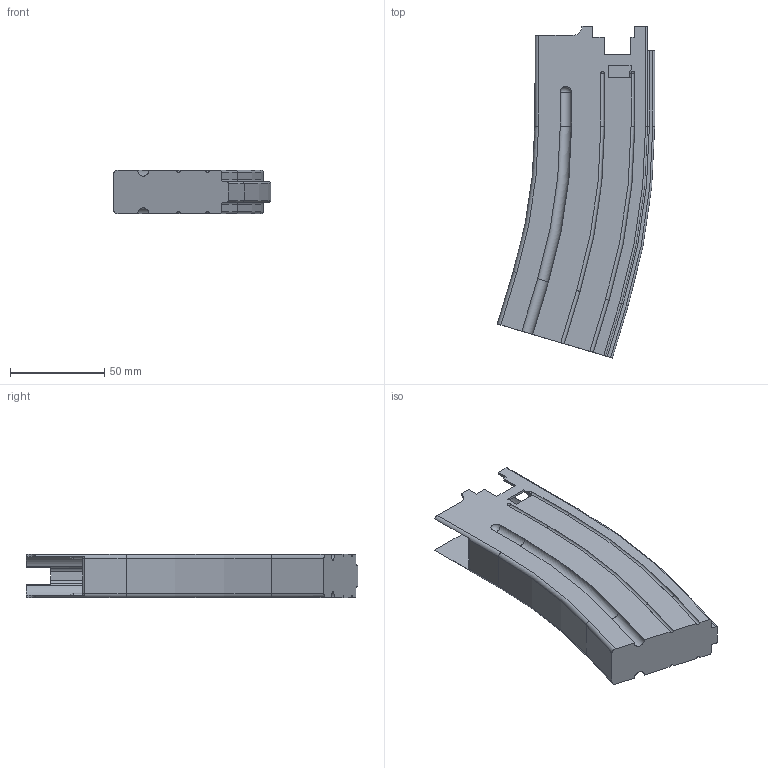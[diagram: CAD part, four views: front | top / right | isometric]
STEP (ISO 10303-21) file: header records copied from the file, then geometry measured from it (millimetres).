
FILE_DESCRIPTION (( 'STEP AP203' ), '1' );
FILE_NAME ('mag.STEP', '2021-12-29T04:18:24', ( '' ), ( '' ), 'SwSTEP 2.0', 'SolidWorks 2015', '' );
FILE_SCHEMA (( 'CONFIG_CONTROL_DESIGN' ));
Length unit declared in the file: millimetre
Products named in the file (1): mag
Bounding box: 83.3 x 175.77 x 22.8 mm (x, y, z)
Volume: 159633.8 mm3; surface area: 39326.7 mm2
Topology: 1 solids, 1 shells, 147 faces, 431 edges, 272 vertices
Faces by surface type: cylinder 54, plane 49, torus 32, sphere 12
Entity records: 5008 total; most frequent: CARTESIAN_POINT 1135, DIRECTION 815, ORIENTED_EDGE 814, EDGE_CURVE 407, AXIS2_PLACEMENT_3D 298, VERTEX_POINT 260, LINE 219, VECTOR 219
